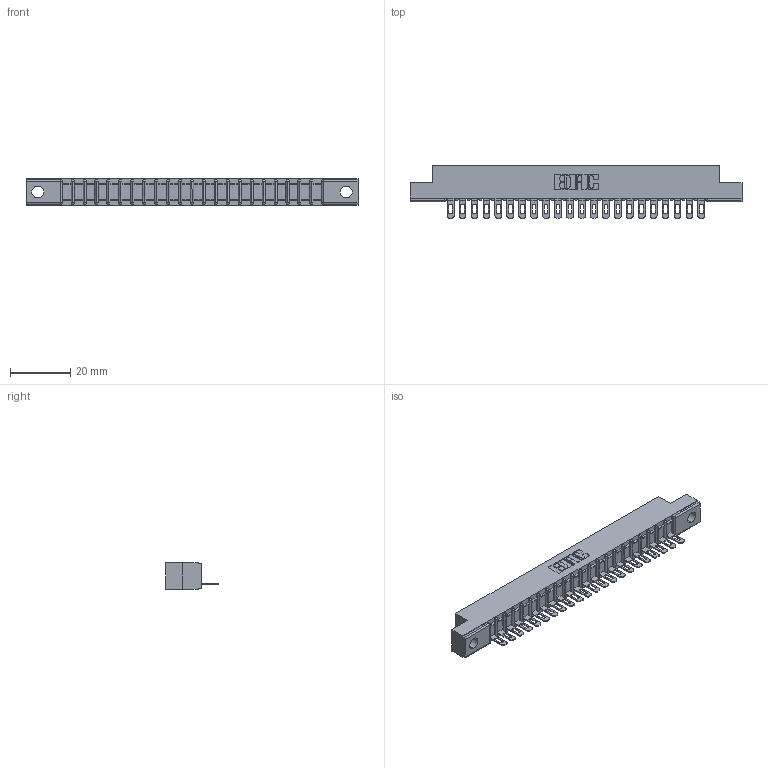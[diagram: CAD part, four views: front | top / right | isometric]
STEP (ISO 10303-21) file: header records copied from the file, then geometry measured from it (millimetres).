
FILE_DESCRIPTION (( 'STEP AP203' ), '1' );
FILE_NAME ('357-022-501-104.STEP', '2019-09-16T23:03:47', ( '' ), ( '' ), 'SwSTEP 2.0', 'SolidWorks 2016', '' );
FILE_SCHEMA (( 'CONFIG_CONTROL_DESIGN' ));
Length unit declared in the file: inch
Products named in the file (3): 357-022-501-104; 307-290-002_501; 307 Part_.156 Dia Mounting Holes
Assembly tree (23 placements, depth 2):
  357-022-501-104
    307 Part_.156 Dia Mounting Holes
    307-290-002_501  x22
Bounding box: 110.19 x 17.42 x 8.71 mm (x, y, z)
Volume: 7187.4 mm3; surface area: 13111.6 mm2
Topology: 23 solids, 23 shells, 1827 faces, 5595 edges, 3666 vertices
Faces by surface type: plane 1052, cylinder 729, sphere 46
Entity records: 22538 total; most frequent: CARTESIAN_POINT 3802, ORIENTED_EDGE 3790, DIRECTION 3699, EDGE_CURVE 1895, LINE 1445, VECTOR 1445, VERTEX_POINT 1230, AXIS2_PLACEMENT_3D 1127
